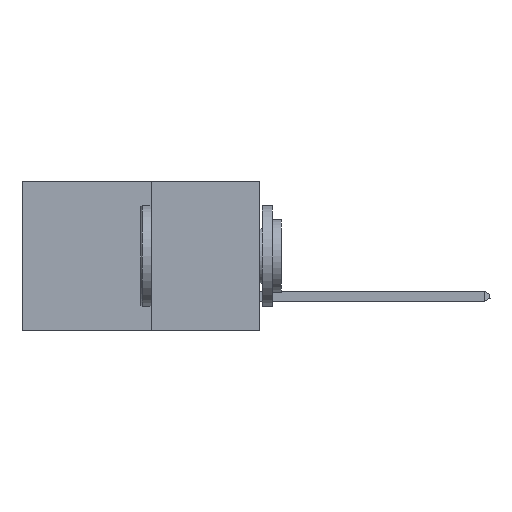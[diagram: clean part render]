
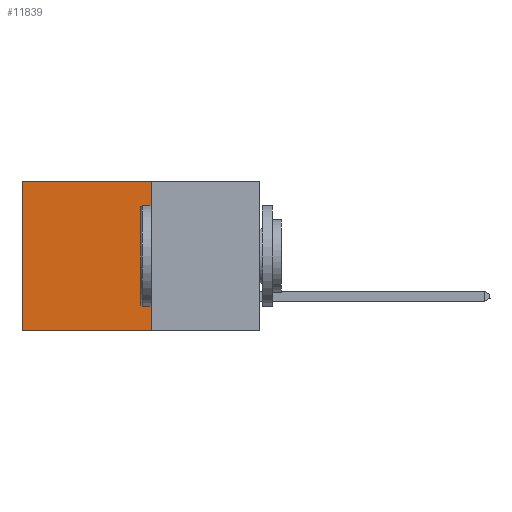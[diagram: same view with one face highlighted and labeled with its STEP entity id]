
A CAD part, left-side view. The second image highlights one B-rep face of the part: STEP entity #11839.
In plain terms, the highlighted planar face has unit normal (-1, 0, 0).
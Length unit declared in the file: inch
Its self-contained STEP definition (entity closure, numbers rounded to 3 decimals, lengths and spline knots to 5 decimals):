
#289 = FACE_OUTER_BOUND ( 'NONE', #15065, .T. ) ;
#343 = ORIENTED_EDGE ( 'NONE', *, *, #4915, .F. ) ;
#693 = ORIENTED_EDGE ( 'NONE', *, *, #10703, .F. ) ;
#1089 = DIRECTION ( 'NONE',  ( 0., 1., 0. ) ) ;
#3046 = VERTEX_POINT ( 'NONE', #4458 ) ;
#3325 = EDGE_CURVE ( 'NONE', #3046, #9393, #17231, .T. ) ;
#3440 = VECTOR ( 'NONE', #18443, 39.37008 ) ;
#3940 = ORIENTED_EDGE ( 'NONE', *, *, #3325, .T. ) ;
#4458 = CARTESIAN_POINT ( 'NONE',  ( 0.277, 0.59, 0. ) ) ;
#4519 = VECTOR ( 'NONE', #13465, 39.37008 ) ;
#4915 = EDGE_CURVE ( 'NONE', #13346, #7227, #16652, .T. ) ;
#5811 = LINE ( 'NONE', #20937, #14414 ) ;
#7207 = CARTESIAN_POINT ( 'NONE',  ( 0.277, 0.59, -0.37 ) ) ;
#7227 = VERTEX_POINT ( 'NONE', #13051 ) ;
#8428 = DIRECTION ( 'NONE',  ( 1., 0., 0. ) ) ;
#9393 = VERTEX_POINT ( 'NONE', #7207 ) ;
#9720 = CARTESIAN_POINT ( 'NONE',  ( 0.277, 0.27, 0. ) ) ;
#10703 = EDGE_CURVE ( 'NONE', #7227, #9393, #5811, .T. ) ;
#11839 = ADVANCED_FACE ( 'NONE', ( #289 ), #18795, .F. ) ;
#12327 = DIRECTION ( 'NONE',  ( 0., 1., 0. ) ) ;
#13051 = CARTESIAN_POINT ( 'NONE',  ( 0.277, 0.27, -0.37 ) ) ;
#13346 = VERTEX_POINT ( 'NONE', #16256 ) ;
#13418 = CARTESIAN_POINT ( 'NONE',  ( 0.277, 0.27, -0.37 ) ) ;
#13465 = DIRECTION ( 'NONE',  ( 0., 0., -1. ) ) ;
#13657 = AXIS2_PLACEMENT_3D ( 'NONE', #15294, #8428, #20498 ) ;
#14414 = VECTOR ( 'NONE', #12327, 39.37008 ) ;
#15040 = ORIENTED_EDGE ( 'NONE', *, *, #18684, .T. ) ;
#15065 = EDGE_LOOP ( 'NONE', ( #3940, #693, #343, #15040 ) ) ;
#15294 = CARTESIAN_POINT ( 'NONE',  ( 0.277, 0.27, -0.37 ) ) ;
#16256 = CARTESIAN_POINT ( 'NONE',  ( 0.277, 0.27, 0. ) ) ;
#16652 = LINE ( 'NONE', #13418, #4519 ) ;
#17231 = LINE ( 'NONE', #18509, #3440 ) ;
#18443 = DIRECTION ( 'NONE',  ( 0., 0., -1. ) ) ;
#18509 = CARTESIAN_POINT ( 'NONE',  ( 0.277, 0.59, -0.37 ) ) ;
#18684 = EDGE_CURVE ( 'NONE', #13346, #3046, #20243, .T. ) ;
#18795 = PLANE ( 'NONE',  #13657 ) ;
#19175 = VECTOR ( 'NONE', #1089, 39.37008 ) ;
#20243 = LINE ( 'NONE', #9720, #19175 ) ;
#20498 = DIRECTION ( 'NONE',  ( 0., 0., -1. ) ) ;
#20937 = CARTESIAN_POINT ( 'NONE',  ( 0.277, 0.27, -0.37 ) ) ;
